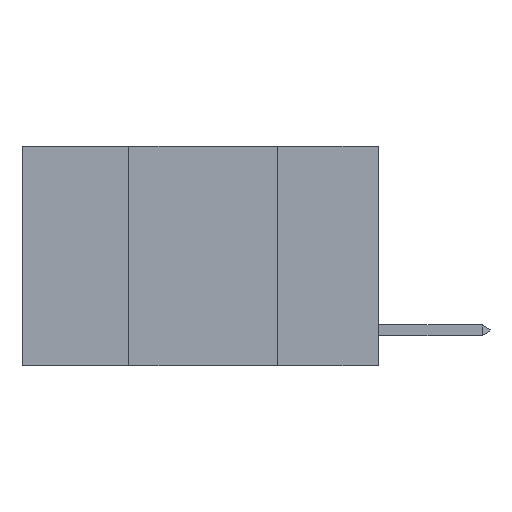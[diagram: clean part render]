
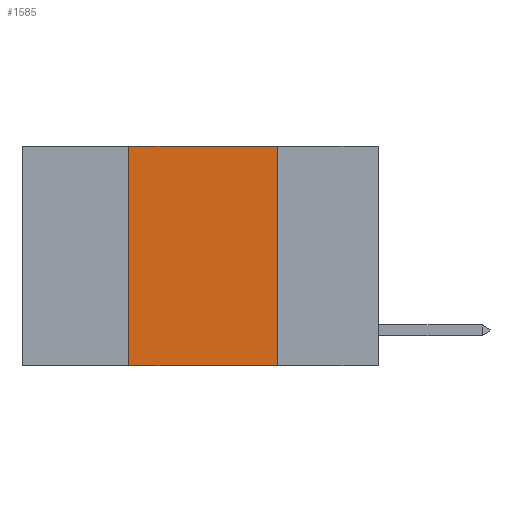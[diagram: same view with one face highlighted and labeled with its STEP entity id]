
A CAD part, left-side view. The second image highlights one B-rep face of the part: STEP entity #1585.
In plain terms, the highlighted planar face has unit normal (-1, 0, 0).
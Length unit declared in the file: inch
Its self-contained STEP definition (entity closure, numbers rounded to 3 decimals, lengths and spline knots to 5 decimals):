
#737 = VERTEX_POINT ( 'NONE', #11610 ) ;
#775 = CARTESIAN_POINT ( 'NONE',  ( 0., 0.17, 0. ) ) ;
#1263 = ORIENTED_EDGE ( 'NONE', *, *, #11340, .F. ) ;
#1585 = ADVANCED_FACE ( 'NONE', ( #8785 ), #13957, .F. ) ;
#2034 = DIRECTION ( 'NONE',  ( 0., -1., 0. ) ) ;
#2133 = CARTESIAN_POINT ( 'NONE',  ( 0., 0.17, 0. ) ) ;
#3413 = VECTOR ( 'NONE', #16604, 39.37008 ) ;
#3425 = DIRECTION ( 'NONE',  ( 1., 0., 0. ) ) ;
#3539 = VECTOR ( 'NONE', #2034, 39.37008 ) ;
#4933 = LINE ( 'NONE', #6927, #18388 ) ;
#5421 = DIRECTION ( 'NONE',  ( 0., 0., 1. ) ) ;
#6927 = CARTESIAN_POINT ( 'NONE',  ( 0., 0.6, -0.37 ) ) ;
#8127 = AXIS2_PLACEMENT_3D ( 'NONE', #22523, #3425, #15731 ) ;
#8638 = LINE ( 'NONE', #775, #3413 ) ;
#8745 = LINE ( 'NONE', #10767, #3539 ) ;
#8785 = FACE_OUTER_BOUND ( 'NONE', #21303, .T. ) ;
#10569 = ORIENTED_EDGE ( 'NONE', *, *, #14139, .T. ) ;
#10767 = CARTESIAN_POINT ( 'NONE',  ( 0., 0.6, 0. ) ) ;
#10881 = EDGE_CURVE ( 'NONE', #19327, #19349, #8638, .T. ) ;
#11340 = EDGE_CURVE ( 'NONE', #18061, #737, #21987, .T. ) ;
#11610 = CARTESIAN_POINT ( 'NONE',  ( 0., 0.42, 0. ) ) ;
#12710 = CARTESIAN_POINT ( 'NONE',  ( 0., 0.42, -0.37 ) ) ;
#13619 = ORIENTED_EDGE ( 'NONE', *, *, #10881, .F. ) ;
#13913 = DIRECTION ( 'NONE',  ( 0., -1., 0. ) ) ;
#13957 = PLANE ( 'NONE',  #8127 ) ;
#14139 = EDGE_CURVE ( 'NONE', #18061, #19349, #4933, .T. ) ;
#15731 = DIRECTION ( 'NONE',  ( 0., 0., -1. ) ) ;
#15962 = CARTESIAN_POINT ( 'NONE',  ( 0., 0.42, 0. ) ) ;
#16604 = DIRECTION ( 'NONE',  ( 0., 0., -1. ) ) ;
#17413 = VECTOR ( 'NONE', #5421, 39.37008 ) ;
#18061 = VERTEX_POINT ( 'NONE', #12710 ) ;
#18388 = VECTOR ( 'NONE', #13913, 39.37008 ) ;
#19327 = VERTEX_POINT ( 'NONE', #2133 ) ;
#19332 = ORIENTED_EDGE ( 'NONE', *, *, #19941, .F. ) ;
#19349 = VERTEX_POINT ( 'NONE', #21473 ) ;
#19941 = EDGE_CURVE ( 'NONE', #737, #19327, #8745, .T. ) ;
#21303 = EDGE_LOOP ( 'NONE', ( #13619, #19332, #1263, #10569 ) ) ;
#21473 = CARTESIAN_POINT ( 'NONE',  ( 0., 0.17, -0.37 ) ) ;
#21987 = LINE ( 'NONE', #15962, #17413 ) ;
#22523 = CARTESIAN_POINT ( 'NONE',  ( 0., 0.6, 0. ) ) ;
